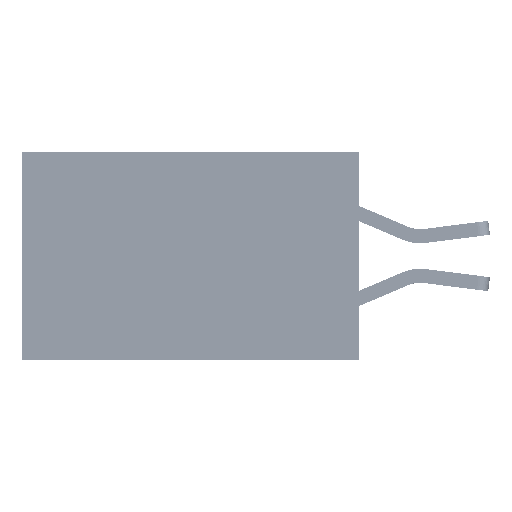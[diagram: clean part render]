
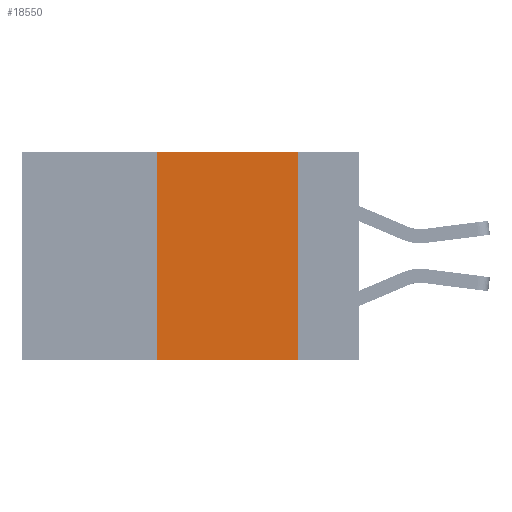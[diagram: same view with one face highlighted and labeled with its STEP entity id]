
A CAD part, left-side view. The second image highlights one B-rep face of the part: STEP entity #18550.
In plain terms, the highlighted planar face has unit normal (-1, 0, 0).
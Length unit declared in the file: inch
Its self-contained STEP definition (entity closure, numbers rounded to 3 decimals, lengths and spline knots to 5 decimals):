
#723 = LINE ( 'NONE', #7479, #19467 ) ;
#1085 = ORIENTED_EDGE ( 'NONE', *, *, #48533, .T. ) ;
#2793 = VECTOR ( 'NONE', #48234, 39.37008 ) ;
#6646 = VERTEX_POINT ( 'NONE', #35767 ) ;
#7479 = CARTESIAN_POINT ( 'NONE',  ( 0., 0.11, 0. ) ) ;
#9718 = LINE ( 'NONE', #27829, #24296 ) ;
#14476 = CARTESIAN_POINT ( 'NONE',  ( 0., 0.36, -0.37 ) ) ;
#14874 = ORIENTED_EDGE ( 'NONE', *, *, #30509, .F. ) ;
#14897 = CARTESIAN_POINT ( 'NONE',  ( 0., 0.6, 0. ) ) ;
#18550 = ADVANCED_FACE ( 'NONE', ( #29615 ), #49537, .F. ) ;
#18804 = DIRECTION ( 'NONE',  ( 0., 0., -1. ) ) ;
#19467 = VECTOR ( 'NONE', #39014, 39.37008 ) ;
#19946 = DIRECTION ( 'NONE',  ( 0., -1., 0. ) ) ;
#20271 = EDGE_LOOP ( 'NONE', ( #33204, #14874, #44715, #1085 ) ) ;
#20454 = CARTESIAN_POINT ( 'NONE',  ( 0., 0.6, 0. ) ) ;
#21684 = CARTESIAN_POINT ( 'NONE',  ( 0., 0.36, 0. ) ) ;
#23220 = VECTOR ( 'NONE', #19946, 39.37008 ) ;
#24296 = VECTOR ( 'NONE', #31892, 39.37008 ) ;
#27829 = CARTESIAN_POINT ( 'NONE',  ( 0., 0.6, -0.37 ) ) ;
#29615 = FACE_OUTER_BOUND ( 'NONE', #20271, .T. ) ;
#30509 = EDGE_CURVE ( 'NONE', #38243, #6646, #34741, .T. ) ;
#31892 = DIRECTION ( 'NONE',  ( 0., -1., 0. ) ) ;
#33204 = ORIENTED_EDGE ( 'NONE', *, *, #41117, .F. ) ;
#34741 = LINE ( 'NONE', #20454, #23220 ) ;
#35767 = CARTESIAN_POINT ( 'NONE',  ( 0., 0.11, 0. ) ) ;
#35861 = VERTEX_POINT ( 'NONE', #46460 ) ;
#38243 = VERTEX_POINT ( 'NONE', #21684 ) ;
#39014 = DIRECTION ( 'NONE',  ( 0., 0., -1. ) ) ;
#39285 = EDGE_CURVE ( 'NONE', #43391, #38243, #45853, .T. ) ;
#41117 = EDGE_CURVE ( 'NONE', #6646, #35861, #723, .T. ) ;
#43391 = VERTEX_POINT ( 'NONE', #14476 ) ;
#44715 = ORIENTED_EDGE ( 'NONE', *, *, #39285, .F. ) ;
#45016 = CARTESIAN_POINT ( 'NONE',  ( 0., 0.36, 0. ) ) ;
#45853 = LINE ( 'NONE', #45016, #2793 ) ;
#46460 = CARTESIAN_POINT ( 'NONE',  ( 0., 0.11, -0.37 ) ) ;
#48234 = DIRECTION ( 'NONE',  ( 0., 0., 1. ) ) ;
#48533 = EDGE_CURVE ( 'NONE', #43391, #35861, #9718, .T. ) ;
#48924 = AXIS2_PLACEMENT_3D ( 'NONE', #14897, #49702, #18804 ) ;
#49537 = PLANE ( 'NONE',  #48924 ) ;
#49702 = DIRECTION ( 'NONE',  ( 1., 0., 0. ) ) ;
